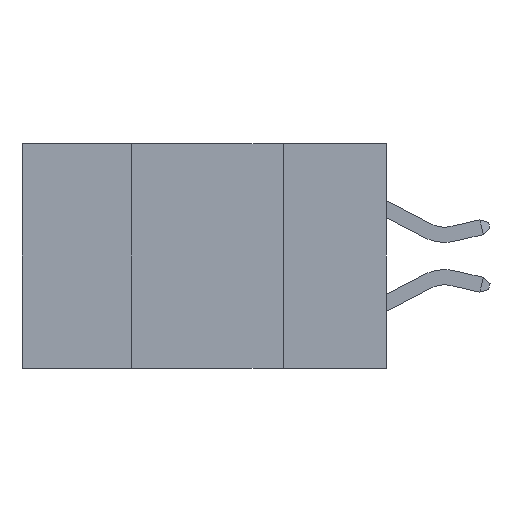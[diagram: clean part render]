
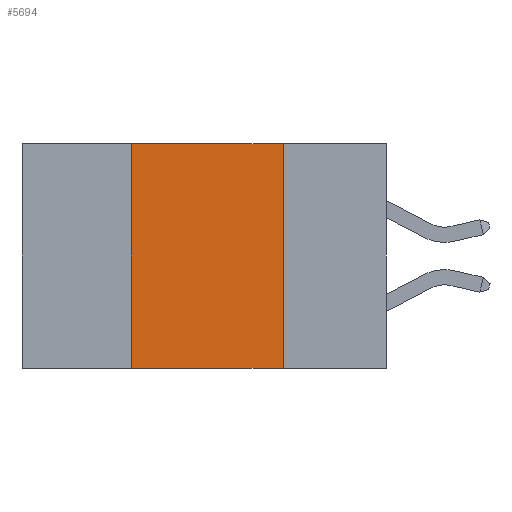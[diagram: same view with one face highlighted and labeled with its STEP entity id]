
A CAD part, left-side view. The second image highlights one B-rep face of the part: STEP entity #5694.
In plain terms, the highlighted planar face has unit normal (-1, 0, 0).
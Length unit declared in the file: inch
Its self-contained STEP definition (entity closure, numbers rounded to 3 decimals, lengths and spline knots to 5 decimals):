
#984 = PLANE ( 'NONE',  #2830 ) ;
#991 = VERTEX_POINT ( 'NONE', #3419 ) ;
#1221 = LINE ( 'NONE', #8068, #7006 ) ;
#1327 = DIRECTION ( 'NONE',  ( 0., -1., 0. ) ) ;
#1813 = EDGE_CURVE ( 'NONE', #9551, #8204, #2119, .T. ) ;
#1977 = VERTEX_POINT ( 'NONE', #4384 ) ;
#2119 = LINE ( 'NONE', #2695, #7764 ) ;
#2400 = CARTESIAN_POINT ( 'NONE',  ( 0., 0.17, 0. ) ) ;
#2695 = CARTESIAN_POINT ( 'NONE',  ( 0., 0.17, 0. ) ) ;
#2740 = DIRECTION ( 'NONE',  ( 0., 0., 1. ) ) ;
#2830 = AXIS2_PLACEMENT_3D ( 'NONE', #7410, #7374, #2980 ) ;
#2980 = DIRECTION ( 'NONE',  ( 0., 0., -1. ) ) ;
#3241 = ORIENTED_EDGE ( 'NONE', *, *, #8083, .T. ) ;
#3417 = ORIENTED_EDGE ( 'NONE', *, *, #4787, .F. ) ;
#3419 = CARTESIAN_POINT ( 'NONE',  ( 0., 0.42, 0. ) ) ;
#4286 = LINE ( 'NONE', #7263, #6648 ) ;
#4384 = CARTESIAN_POINT ( 'NONE',  ( 0., 0.42, -0.37 ) ) ;
#4787 = EDGE_CURVE ( 'NONE', #1977, #991, #4286, .T. ) ;
#4795 = EDGE_CURVE ( 'NONE', #991, #9551, #1221, .T. ) ;
#5314 = ORIENTED_EDGE ( 'NONE', *, *, #4795, .F. ) ;
#5694 = ADVANCED_FACE ( 'NONE', ( #9423 ), #984, .F. ) ;
#5803 = DIRECTION ( 'NONE',  ( 0., 0., -1. ) ) ;
#6515 = ORIENTED_EDGE ( 'NONE', *, *, #1813, .F. ) ;
#6600 = LINE ( 'NONE', #7917, #6833 ) ;
#6629 = CARTESIAN_POINT ( 'NONE',  ( 0., 0.17, -0.37 ) ) ;
#6648 = VECTOR ( 'NONE', #2740, 39.37008 ) ;
#6833 = VECTOR ( 'NONE', #9383, 39.37008 ) ;
#7006 = VECTOR ( 'NONE', #1327, 39.37008 ) ;
#7263 = CARTESIAN_POINT ( 'NONE',  ( 0., 0.42, 0. ) ) ;
#7374 = DIRECTION ( 'NONE',  ( 1., 0., 0. ) ) ;
#7410 = CARTESIAN_POINT ( 'NONE',  ( 0., 0.6, 0. ) ) ;
#7764 = VECTOR ( 'NONE', #5803, 39.37008 ) ;
#7917 = CARTESIAN_POINT ( 'NONE',  ( 0., 0.6, -0.37 ) ) ;
#8068 = CARTESIAN_POINT ( 'NONE',  ( 0., 0.6, 0. ) ) ;
#8083 = EDGE_CURVE ( 'NONE', #1977, #8204, #6600, .T. ) ;
#8204 = VERTEX_POINT ( 'NONE', #6629 ) ;
#8629 = EDGE_LOOP ( 'NONE', ( #6515, #5314, #3417, #3241 ) ) ;
#9383 = DIRECTION ( 'NONE',  ( 0., -1., 0. ) ) ;
#9423 = FACE_OUTER_BOUND ( 'NONE', #8629, .T. ) ;
#9551 = VERTEX_POINT ( 'NONE', #2400 ) ;
